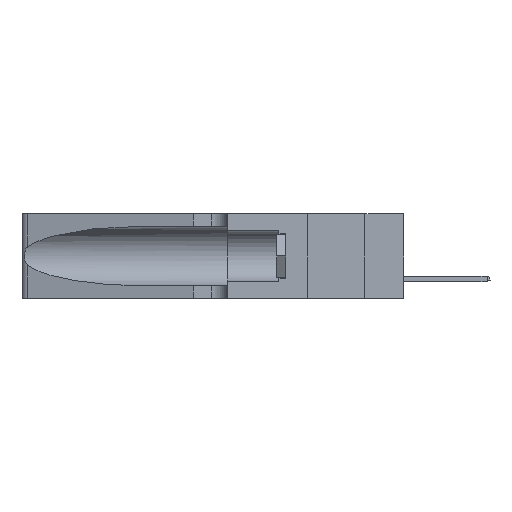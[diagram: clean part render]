
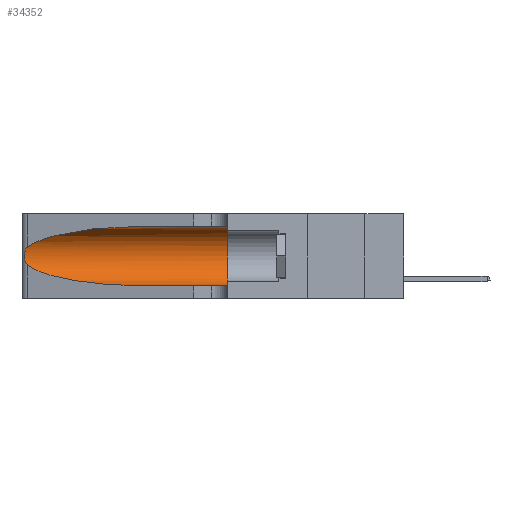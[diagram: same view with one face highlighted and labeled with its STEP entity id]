
A CAD part, left-side view. The second image highlights one B-rep face of the part: STEP entity #34352.
In plain terms, the highlighted cylindrical face has radius 3.308 mm (diameter 6.617 mm), a partial arc.
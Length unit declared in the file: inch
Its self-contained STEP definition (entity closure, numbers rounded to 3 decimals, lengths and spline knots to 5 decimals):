
#1034 =( BOUNDED_CURVE ( )  B_SPLINE_CURVE ( 3, ( #4039, #33065, #33213, #27037 ),
 .UNSPECIFIED., .F., .T. ) 
 B_SPLINE_CURVE_WITH_KNOTS ( ( 4, 4 ),
 ( 3.44316, 4.71239 ),
 .UNSPECIFIED. ) 
 CURVE ( )  GEOMETRIC_REPRESENTATION_ITEM ( )  RATIONAL_B_SPLINE_CURVE ( ( 1., 0.87, 0.87, 1. ) ) 
 REPRESENTATION_ITEM ( '' )  );
#1132 = CARTESIAN_POINT ( 'NONE',  ( 0.26075, 1.23896, 0.19203 ) ) ;
#1282 = CARTESIAN_POINT ( 'NONE',  ( 0.25856, 1.23593, 0.16098 ) ) ;
#1317 = DIRECTION ( 'NONE',  ( 0., 0., 1. ) ) ;
#1424 = CARTESIAN_POINT ( 'NONE',  ( 0.25487, 1.22718, 0.22369 ) ) ;
#1550 = EDGE_CURVE ( 'NONE', #28175, #20397, #33434, .T. ) ;
#2980 = VERTEX_POINT ( 'NONE', #6709 ) ;
#3837 = ORIENTED_EDGE ( 'NONE', *, *, #27459, .T. ) ;
#4039 = CARTESIAN_POINT ( 'NONE',  ( 0.25487, 1.22718, 0.14631 ) ) ;
#4559 = CARTESIAN_POINT ( 'NONE',  ( 0.25639, 1.23186, 0.15144 ) ) ;
#6563 = VERTEX_POINT ( 'NONE', #10037 ) ;
#6709 = CARTESIAN_POINT ( 'NONE',  ( 0.25487, 1.22718, 0.14631 ) ) ;
#7121 = ORIENTED_EDGE ( 'NONE', *, *, #37485, .T. ) ;
#7285 = ORIENTED_EDGE ( 'NONE', *, *, #28361, .F. ) ;
#7816 = LINE ( 'NONE', #36872, #24301 ) ;
#7994 = CARTESIAN_POINT ( 'NONE',  ( 0.25789, 1.23486, 0.15765 ) ) ;
#9165 = CARTESIAN_POINT ( 'NONE',  ( 0.1305, 1.61858, 0.185 ) ) ;
#10037 = CARTESIAN_POINT ( 'NONE',  ( 0.1305, 0.72297, 0.05475 ) ) ;
#11144 = CARTESIAN_POINT ( 'NONE',  ( 0.25787, 1.23484, 0.2124 ) ) ;
#11583 = CARTESIAN_POINT ( 'NONE',  ( 0.25555, 1.22993, 0.14849 ) ) ;
#12324 = DIRECTION ( 'NONE',  ( 0., 0., -1. ) ) ;
#13153 = VECTOR ( 'NONE', #19328, 39.37008 ) ;
#13357 = CIRCLE ( 'NONE', #21643, 0.13025 ) ;
#14359 = CYLINDRICAL_SURFACE ( 'NONE', #17831, 0.13025 ) ;
#14388 = CARTESIAN_POINT ( 'NONE',  ( 0.1305, 0.35, 0.31525 ) ) ;
#14614 = CARTESIAN_POINT ( 'NONE',  ( 0.25555, 1.22994, 0.2215 ) ) ;
#15890 = EDGE_CURVE ( 'NONE', #22235, #21091, #13357, .T. ) ;
#16846 = B_SPLINE_CURVE_WITH_KNOTS ( 'NONE', 3,
 ( #1424, #14614, #20959, #11144, #21254, #21405, #1132, #18225, #34186, #1282, #7994, #4559, #11583, #37631 ),
 .UNSPECIFIED., .F., .F.,
 ( 4, 2, 2, 2, 2, 2, 4 ),
 ( 0., 0.00027, 0.00053, 0.00107, 0.0016, 0.00187, 0.00214 ),
 .UNSPECIFIED. ) ;
#16976 = DIRECTION ( 'NONE',  ( 0., 1., 0. ) ) ;
#17159 = DIRECTION ( 'NONE',  ( 0., -1., 0. ) ) ;
#17688 = CARTESIAN_POINT ( 'NONE',  ( 0.1305, 0.35, 0.185 ) ) ;
#17831 = AXIS2_PLACEMENT_3D ( 'NONE', #9165, #35208, #12324 ) ;
#18225 = CARTESIAN_POINT ( 'NONE',  ( 0.26075, 1.23896, 0.178 ) ) ;
#19328 = DIRECTION ( 'NONE',  ( 0., -1., 0. ) ) ;
#20314 = ORIENTED_EDGE ( 'NONE', *, *, #39994, .T. ) ;
#20397 = VERTEX_POINT ( 'NONE', #28045 ) ;
#20959 = CARTESIAN_POINT ( 'NONE',  ( 0.25639, 1.23184, 0.21858 ) ) ;
#21091 = VERTEX_POINT ( 'NONE', #38175 ) ;
#21254 = CARTESIAN_POINT ( 'NONE',  ( 0.25854, 1.2359, 0.20912 ) ) ;
#21405 = CARTESIAN_POINT ( 'NONE',  ( 0.26018, 1.23835, 0.19895 ) ) ;
#21643 = AXIS2_PLACEMENT_3D ( 'NONE', #17688, #16976, #1317 ) ;
#22235 = VERTEX_POINT ( 'NONE', #14388 ) ;
#22481 = CARTESIAN_POINT ( 'NONE',  ( 0.1305, 1.61858, 0.31525 ) ) ;
#24301 = VECTOR ( 'NONE', #17159, 39.37008 ) ;
#26040 = LINE ( 'NONE', #22481, #13153 ) ;
#27037 = CARTESIAN_POINT ( 'NONE',  ( 0.1305, 0.72297, 0.05475 ) ) ;
#27459 = EDGE_CURVE ( 'NONE', #20397, #2980, #16846, .T. ) ;
#28045 = CARTESIAN_POINT ( 'NONE',  ( 0.25487, 1.22718, 0.22369 ) ) ;
#28175 = VERTEX_POINT ( 'NONE', #34414 ) ;
#28361 = EDGE_CURVE ( 'NONE', #28175, #22235, #26040, .T. ) ;
#31284 = EDGE_LOOP ( 'NONE', ( #40174, #3837, #7121, #20314, #32835, #7285 ) ) ;
#32835 = ORIENTED_EDGE ( 'NONE', *, *, #15890, .F. ) ;
#33065 = CARTESIAN_POINT ( 'NONE',  ( 0.2373, 1.15595, 0.08982 ) ) ;
#33213 = CARTESIAN_POINT ( 'NONE',  ( 0.18966, 0.96281, 0.05475 ) ) ;
#33434 =( BOUNDED_CURVE ( )  B_SPLINE_CURVE ( 3, ( #35513, #38543, #38251, #41553 ),
 .UNSPECIFIED., .F., .F. ) 
 B_SPLINE_CURVE_WITH_KNOTS ( ( 4, 4 ),
 ( 1.5708, 2.84003 ),
 .UNSPECIFIED. ) 
 CURVE ( )  GEOMETRIC_REPRESENTATION_ITEM ( )  RATIONAL_B_SPLINE_CURVE ( ( 1., 0.87, 0.87, 1. ) ) 
 REPRESENTATION_ITEM ( '' )  );
#33931 = FACE_OUTER_BOUND ( 'NONE', #31284, .T. ) ;
#34186 = CARTESIAN_POINT ( 'NONE',  ( 0.26017, 1.23833, 0.17102 ) ) ;
#34352 = ADVANCED_FACE ( 'NONE', ( #33931 ), #14359, .F. ) ;
#34414 = CARTESIAN_POINT ( 'NONE',  ( 0.1305, 0.72297, 0.31525 ) ) ;
#35208 = DIRECTION ( 'NONE',  ( 0., -1., 0. ) ) ;
#35513 = CARTESIAN_POINT ( 'NONE',  ( 0.1305, 0.72297, 0.31525 ) ) ;
#36872 = CARTESIAN_POINT ( 'NONE',  ( 0.1305, 1.61858, 0.05475 ) ) ;
#37485 = EDGE_CURVE ( 'NONE', #2980, #6563, #1034, .T. ) ;
#37631 = CARTESIAN_POINT ( 'NONE',  ( 0.25487, 1.22718, 0.14631 ) ) ;
#38175 = CARTESIAN_POINT ( 'NONE',  ( 0.1305, 0.35, 0.05475 ) ) ;
#38251 = CARTESIAN_POINT ( 'NONE',  ( 0.2373, 1.15595, 0.28018 ) ) ;
#38543 = CARTESIAN_POINT ( 'NONE',  ( 0.18966, 0.96281, 0.31525 ) ) ;
#39994 = EDGE_CURVE ( 'NONE', #6563, #21091, #7816, .T. ) ;
#40174 = ORIENTED_EDGE ( 'NONE', *, *, #1550, .T. ) ;
#41553 = CARTESIAN_POINT ( 'NONE',  ( 0.25487, 1.22718, 0.22369 ) ) ;
